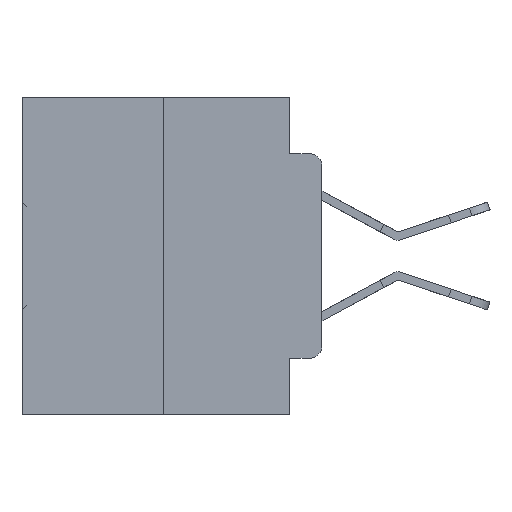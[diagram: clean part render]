
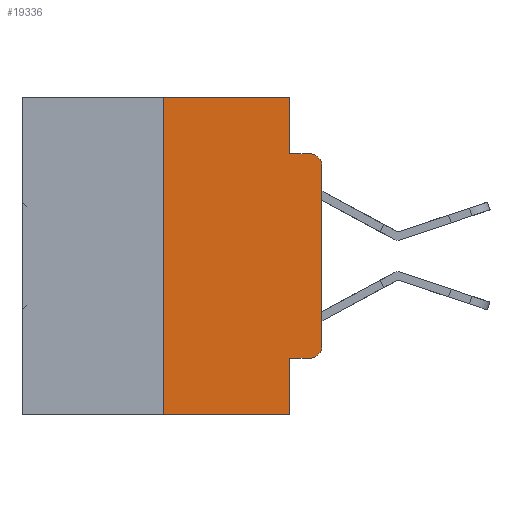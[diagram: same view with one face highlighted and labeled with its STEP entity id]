
A CAD part, left-side view. The second image highlights one B-rep face of the part: STEP entity #19336.
In plain terms, the highlighted planar face has unit normal (-1, 0, 0).
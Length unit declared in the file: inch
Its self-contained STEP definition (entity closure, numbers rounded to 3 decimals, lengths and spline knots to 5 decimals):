
#208 = DIRECTION ( 'NONE',  ( 0., 0., 1. ) ) ;
#368 = VECTOR ( 'NONE', #34608, 39.37008 ) ;
#460 = CARTESIAN_POINT ( 'NONE',  ( 0., 0.02, -0.0885 ) ) ;
#1144 = CIRCLE ( 'NONE', #27971, 0.02 ) ;
#1451 = DIRECTION ( 'NONE',  ( 0., 0., -1. ) ) ;
#1798 = DIRECTION ( 'NONE',  ( 0., -1., 0. ) ) ;
#3814 = CARTESIAN_POINT ( 'NONE',  ( 0., 0.051, 0. ) ) ;
#4881 = EDGE_CURVE ( 'NONE', #33472, #18927, #17386, .T. ) ;
#5960 = LINE ( 'NONE', #17113, #34369 ) ;
#7114 = CARTESIAN_POINT ( 'NONE',  ( 0., 0., -0.1085 ) ) ;
#7481 = CARTESIAN_POINT ( 'NONE',  ( 0., 0.473, 0. ) ) ;
#7519 = CARTESIAN_POINT ( 'NONE',  ( 0., 0.051, -0.5 ) ) ;
#7977 = CARTESIAN_POINT ( 'NONE',  ( 0., 0.051, -0.4115 ) ) ;
#7989 = VERTEX_POINT ( 'NONE', #27976 ) ;
#8313 = VECTOR ( 'NONE', #13643, 39.37008 ) ;
#8578 = CARTESIAN_POINT ( 'NONE',  ( 0., 0.051, -0.0885 ) ) ;
#8831 = EDGE_CURVE ( 'NONE', #23051, #11306, #5960, .T. ) ;
#9597 = CARTESIAN_POINT ( 'NONE',  ( 0., 0.25, -0.5 ) ) ;
#9602 = ORIENTED_EDGE ( 'NONE', *, *, #30265, .F. ) ;
#9671 = AXIS2_PLACEMENT_3D ( 'NONE', #12480, #12660, #23805 ) ;
#9678 = LINE ( 'NONE', #7481, #28985 ) ;
#10036 = FACE_OUTER_BOUND ( 'NONE', #19059, .T. ) ;
#10407 = EDGE_CURVE ( 'NONE', #33472, #16335, #19801, .T. ) ;
#10940 = EDGE_CURVE ( 'NONE', #7989, #13276, #22307, .T. ) ;
#11261 = EDGE_CURVE ( 'NONE', #11306, #13276, #1144, .T. ) ;
#11306 = VERTEX_POINT ( 'NONE', #7114 ) ;
#11816 = CARTESIAN_POINT ( 'NONE',  ( 0., 0., -0.3915 ) ) ;
#12480 = CARTESIAN_POINT ( 'NONE',  ( 0., 0.02, -0.3915 ) ) ;
#12660 = DIRECTION ( 'NONE',  ( -1., 0., 0. ) ) ;
#12814 = ORIENTED_EDGE ( 'NONE', *, *, #10940, .F. ) ;
#13035 = EDGE_CURVE ( 'NONE', #21196, #21367, #18781, .T. ) ;
#13135 = CARTESIAN_POINT ( 'NONE',  ( 0., 0.02, -0.1085 ) ) ;
#13276 = VERTEX_POINT ( 'NONE', #460 ) ;
#13643 = DIRECTION ( 'NONE',  ( 0., -1., 0. ) ) ;
#13743 = VECTOR ( 'NONE', #17555, 39.37008 ) ;
#15107 = ORIENTED_EDGE ( 'NONE', *, *, #13035, .T. ) ;
#15711 = DIRECTION ( 'NONE',  ( -1., 0., 0. ) ) ;
#15718 = PLANE ( 'NONE',  #22049 ) ;
#16234 = ORIENTED_EDGE ( 'NONE', *, *, #10407, .F. ) ;
#16335 = VERTEX_POINT ( 'NONE', #28924 ) ;
#16392 = CARTESIAN_POINT ( 'NONE',  ( 0., 0.051, -0.4115 ) ) ;
#17113 = CARTESIAN_POINT ( 'NONE',  ( 0., 0., 0. ) ) ;
#17337 = VERTEX_POINT ( 'NONE', #24293 ) ;
#17386 = LINE ( 'NONE', #25394, #13743 ) ;
#17555 = DIRECTION ( 'NONE',  ( 0., -1., 0. ) ) ;
#17773 = VECTOR ( 'NONE', #32903, 39.37008 ) ;
#18781 = LINE ( 'NONE', #16392, #8313 ) ;
#18927 = VERTEX_POINT ( 'NONE', #7519 ) ;
#19059 = EDGE_LOOP ( 'NONE', ( #23302, #23380, #12814, #9602, #24349, #16234, #24565, #23900, #15107, #20592 ) ) ;
#19080 = CARTESIAN_POINT ( 'NONE',  ( 0., 0.25, 0. ) ) ;
#19255 = EDGE_CURVE ( 'NONE', #16335, #17337, #9678, .T. ) ;
#19336 = ADVANCED_FACE ( 'NONE', ( #10036 ), #15718, .F. ) ;
#19801 = LINE ( 'NONE', #19080, #30527 ) ;
#20592 = ORIENTED_EDGE ( 'NONE', *, *, #33881, .T. ) ;
#21196 = VERTEX_POINT ( 'NONE', #7977 ) ;
#21201 = DIRECTION ( 'NONE',  ( 0., 0., -1. ) ) ;
#21367 = VERTEX_POINT ( 'NONE', #25314 ) ;
#22049 = AXIS2_PLACEMENT_3D ( 'NONE', #26472, #24104, #1451 ) ;
#22307 = LINE ( 'NONE', #8578, #25810 ) ;
#23051 = VERTEX_POINT ( 'NONE', #11816 ) ;
#23302 = ORIENTED_EDGE ( 'NONE', *, *, #8831, .T. ) ;
#23380 = ORIENTED_EDGE ( 'NONE', *, *, #11261, .T. ) ;
#23537 = LINE ( 'NONE', #3814, #368 ) ;
#23805 = DIRECTION ( 'NONE',  ( 0., 0., -1. ) ) ;
#23900 = ORIENTED_EDGE ( 'NONE', *, *, #34882, .F. ) ;
#24104 = DIRECTION ( 'NONE',  ( 1., 0., 0. ) ) ;
#24293 = CARTESIAN_POINT ( 'NONE',  ( 0., 0.051, 0. ) ) ;
#24349 = ORIENTED_EDGE ( 'NONE', *, *, #19255, .F. ) ;
#24565 = ORIENTED_EDGE ( 'NONE', *, *, #4881, .T. ) ;
#25314 = CARTESIAN_POINT ( 'NONE',  ( 0., 0.02, -0.4115 ) ) ;
#25394 = CARTESIAN_POINT ( 'NONE',  ( 0., 0.473, -0.5 ) ) ;
#25417 = CIRCLE ( 'NONE', #9671, 0.02 ) ;
#25810 = VECTOR ( 'NONE', #30110, 39.37008 ) ;
#26472 = CARTESIAN_POINT ( 'NONE',  ( 0., 0.473, 0. ) ) ;
#27458 = LINE ( 'NONE', #29818, #17773 ) ;
#27971 = AXIS2_PLACEMENT_3D ( 'NONE', #13135, #15711, #21201 ) ;
#27976 = CARTESIAN_POINT ( 'NONE',  ( 0., 0.051, -0.0885 ) ) ;
#28924 = CARTESIAN_POINT ( 'NONE',  ( 0., 0.25, 0. ) ) ;
#28985 = VECTOR ( 'NONE', #1798, 39.37008 ) ;
#29818 = CARTESIAN_POINT ( 'NONE',  ( 0., 0.051, 0. ) ) ;
#30110 = DIRECTION ( 'NONE',  ( 0., -1., 0. ) ) ;
#30213 = DIRECTION ( 'NONE',  ( 0., 0., 1. ) ) ;
#30265 = EDGE_CURVE ( 'NONE', #17337, #7989, #27458, .T. ) ;
#30527 = VECTOR ( 'NONE', #208, 39.37008 ) ;
#32903 = DIRECTION ( 'NONE',  ( 0., 0., -1. ) ) ;
#33472 = VERTEX_POINT ( 'NONE', #9597 ) ;
#33881 = EDGE_CURVE ( 'NONE', #21367, #23051, #25417, .T. ) ;
#34369 = VECTOR ( 'NONE', #30213, 39.37008 ) ;
#34608 = DIRECTION ( 'NONE',  ( 0., 0., -1. ) ) ;
#34882 = EDGE_CURVE ( 'NONE', #21196, #18927, #23537, .T. ) ;
